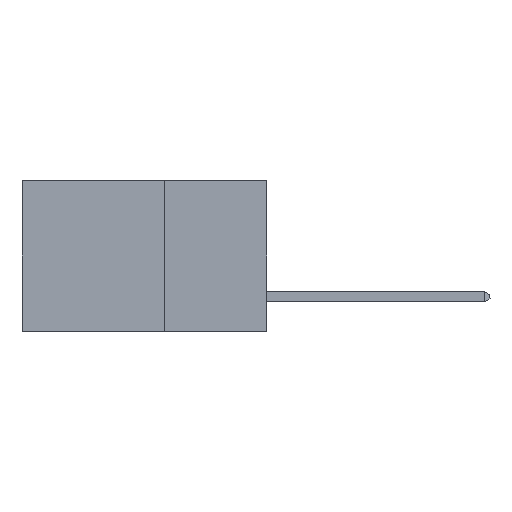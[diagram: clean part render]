
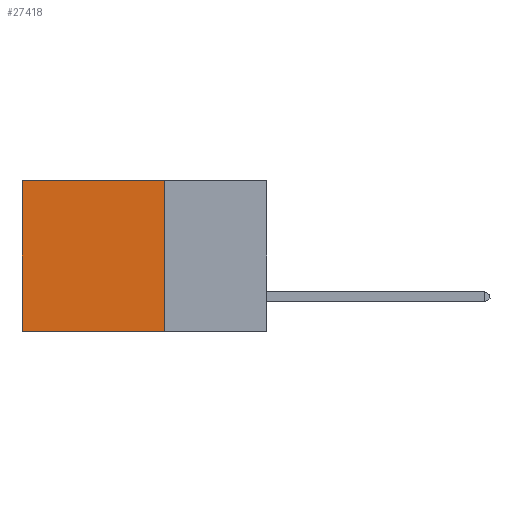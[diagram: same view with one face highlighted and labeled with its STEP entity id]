
A CAD part, left-side view. The second image highlights one B-rep face of the part: STEP entity #27418.
In plain terms, the highlighted planar face has unit normal (-1, 0, 0).
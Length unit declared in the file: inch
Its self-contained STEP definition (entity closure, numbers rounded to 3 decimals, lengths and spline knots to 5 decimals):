
#630 = CARTESIAN_POINT ( 'NONE',  ( 0.2875, 0.25, -0.37 ) ) ;
#1911 = ORIENTED_EDGE ( 'NONE', *, *, #17574, .F. ) ;
#1928 = DIRECTION ( 'NONE',  ( 0., 0., -1. ) ) ;
#2682 = EDGE_CURVE ( 'NONE', #11807, #19245, #29417, .T. ) ;
#2735 = CARTESIAN_POINT ( 'NONE',  ( 0.2875, 0.25, 0. ) ) ;
#3727 = VERTEX_POINT ( 'NONE', #33443 ) ;
#5060 = CARTESIAN_POINT ( 'NONE',  ( 0.2875, 0.6, 0. ) ) ;
#5323 = VECTOR ( 'NONE', #23802, 39.37008 ) ;
#7180 = CARTESIAN_POINT ( 'NONE',  ( 0.2875, 0.25, 0. ) ) ;
#8622 = AXIS2_PLACEMENT_3D ( 'NONE', #7180, #18000, #1928 ) ;
#9549 = VECTOR ( 'NONE', #12150, 39.37008 ) ;
#10317 = CARTESIAN_POINT ( 'NONE',  ( 0.2875, 0.25, 0. ) ) ;
#10819 = CARTESIAN_POINT ( 'NONE',  ( 0.2875, 0.6, -0.37 ) ) ;
#10865 = EDGE_CURVE ( 'NONE', #3727, #19245, #17100, .T. ) ;
#11807 = VERTEX_POINT ( 'NONE', #630 ) ;
#12150 = DIRECTION ( 'NONE',  ( 0., 0., -1. ) ) ;
#12867 = DIRECTION ( 'NONE',  ( 0., 1., 0. ) ) ;
#13028 = DIRECTION ( 'NONE',  ( 0., 1., 0. ) ) ;
#16169 = ORIENTED_EDGE ( 'NONE', *, *, #10865, .T. ) ;
#16594 = EDGE_CURVE ( 'NONE', #25761, #3727, #19510, .T. ) ;
#16722 = LINE ( 'NONE', #17460, #9549 ) ;
#17100 = LINE ( 'NONE', #5060, #5323 ) ;
#17460 = CARTESIAN_POINT ( 'NONE',  ( 0.2875, 0.25, 0. ) ) ;
#17574 = EDGE_CURVE ( 'NONE', #25761, #11807, #16722, .T. ) ;
#18000 = DIRECTION ( 'NONE',  ( 1., 0., 0. ) ) ;
#19245 = VERTEX_POINT ( 'NONE', #10819 ) ;
#19510 = LINE ( 'NONE', #10317, #25745 ) ;
#22339 = VECTOR ( 'NONE', #12867, 39.37008 ) ;
#23519 = CARTESIAN_POINT ( 'NONE',  ( 0.2875, 0.25, -0.37 ) ) ;
#23721 = EDGE_LOOP ( 'NONE', ( #16169, #31566, #1911, #28125 ) ) ;
#23802 = DIRECTION ( 'NONE',  ( 0., 0., -1. ) ) ;
#25745 = VECTOR ( 'NONE', #13028, 39.37008 ) ;
#25761 = VERTEX_POINT ( 'NONE', #2735 ) ;
#27418 = ADVANCED_FACE ( 'NONE', ( #32441 ), #33951, .F. ) ;
#28125 = ORIENTED_EDGE ( 'NONE', *, *, #16594, .T. ) ;
#29417 = LINE ( 'NONE', #23519, #22339 ) ;
#31566 = ORIENTED_EDGE ( 'NONE', *, *, #2682, .F. ) ;
#32441 = FACE_OUTER_BOUND ( 'NONE', #23721, .T. ) ;
#33443 = CARTESIAN_POINT ( 'NONE',  ( 0.2875, 0.6, 0. ) ) ;
#33951 = PLANE ( 'NONE',  #8622 ) ;
